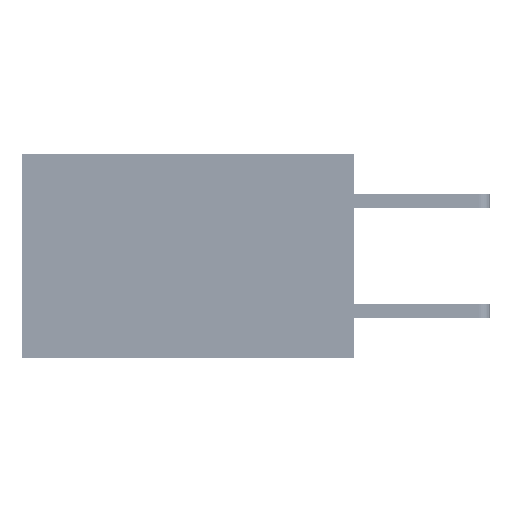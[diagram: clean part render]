
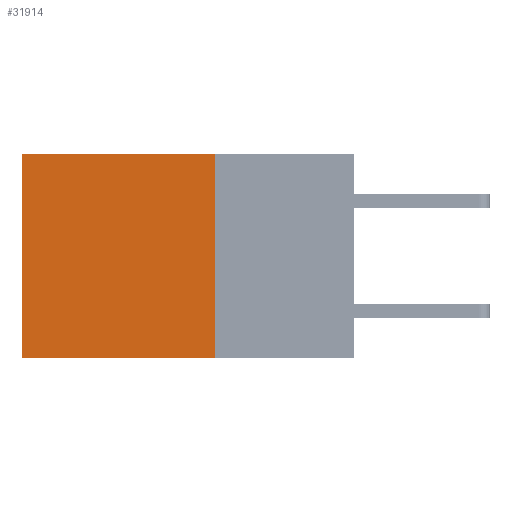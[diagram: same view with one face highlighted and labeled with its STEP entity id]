
A CAD part, left-side view. The second image highlights one B-rep face of the part: STEP entity #31914.
In plain terms, the highlighted planar face has unit normal (-1, 0, 0).
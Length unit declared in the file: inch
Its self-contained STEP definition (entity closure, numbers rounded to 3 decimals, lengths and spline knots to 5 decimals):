
#1111 = VECTOR ( 'NONE', #12336, 39.37008 ) ;
#1145 = LINE ( 'NONE', #8287, #14936 ) ;
#3515 = DIRECTION ( 'NONE',  ( 0., 1., 0. ) ) ;
#4179 = VERTEX_POINT ( 'NONE', #20440 ) ;
#6570 = LINE ( 'NONE', #49297, #46572 ) ;
#6988 = ORIENTED_EDGE ( 'NONE', *, *, #33699, .F. ) ;
#7126 = PLANE ( 'NONE',  #24508 ) ;
#7382 = DIRECTION ( 'NONE',  ( 1., 0., 0. ) ) ;
#7736 = ORIENTED_EDGE ( 'NONE', *, *, #20997, .T. ) ;
#7908 = LINE ( 'NONE', #23696, #30433 ) ;
#8287 = CARTESIAN_POINT ( 'NONE',  ( 0.2875, 0.25, 0. ) ) ;
#12336 = DIRECTION ( 'NONE',  ( 0., 0., -1. ) ) ;
#13899 = CARTESIAN_POINT ( 'NONE',  ( 0.2875, 0.25, -0.37 ) ) ;
#14936 = VECTOR ( 'NONE', #43878, 39.37008 ) ;
#20156 = EDGE_CURVE ( 'NONE', #23077, #30723, #27866, .T. ) ;
#20217 = CARTESIAN_POINT ( 'NONE',  ( 0.2875, 0.25, 0. ) ) ;
#20255 = EDGE_CURVE ( 'NONE', #23077, #25074, #1145, .T. ) ;
#20440 = CARTESIAN_POINT ( 'NONE',  ( 0.2875, 0.6, -0.37 ) ) ;
#20997 = EDGE_CURVE ( 'NONE', #25074, #4179, #7908, .T. ) ;
#21891 = FACE_OUTER_BOUND ( 'NONE', #29704, .T. ) ;
#22675 = ORIENTED_EDGE ( 'NONE', *, *, #20156, .F. ) ;
#23077 = VERTEX_POINT ( 'NONE', #30541 ) ;
#23696 = CARTESIAN_POINT ( 'NONE',  ( 0.2875, 0.6, 0. ) ) ;
#24508 = AXIS2_PLACEMENT_3D ( 'NONE', #42236, #7382, #29523 ) ;
#25074 = VERTEX_POINT ( 'NONE', #44939 ) ;
#27866 = LINE ( 'NONE', #20217, #1111 ) ;
#29523 = DIRECTION ( 'NONE',  ( 0., 0., -1. ) ) ;
#29704 = EDGE_LOOP ( 'NONE', ( #7736, #6988, #22675, #43921 ) ) ;
#30433 = VECTOR ( 'NONE', #43270, 39.37008 ) ;
#30541 = CARTESIAN_POINT ( 'NONE',  ( 0.2875, 0.25, 0. ) ) ;
#30723 = VERTEX_POINT ( 'NONE', #13899 ) ;
#31914 = ADVANCED_FACE ( 'NONE', ( #21891 ), #7126, .F. ) ;
#33699 = EDGE_CURVE ( 'NONE', #30723, #4179, #6570, .T. ) ;
#42236 = CARTESIAN_POINT ( 'NONE',  ( 0.2875, 0.25, 0. ) ) ;
#43270 = DIRECTION ( 'NONE',  ( 0., 0., -1. ) ) ;
#43878 = DIRECTION ( 'NONE',  ( 0., 1., 0. ) ) ;
#43921 = ORIENTED_EDGE ( 'NONE', *, *, #20255, .T. ) ;
#44939 = CARTESIAN_POINT ( 'NONE',  ( 0.2875, 0.6, 0. ) ) ;
#46572 = VECTOR ( 'NONE', #3515, 39.37008 ) ;
#49297 = CARTESIAN_POINT ( 'NONE',  ( 0.2875, 0.25, -0.37 ) ) ;
